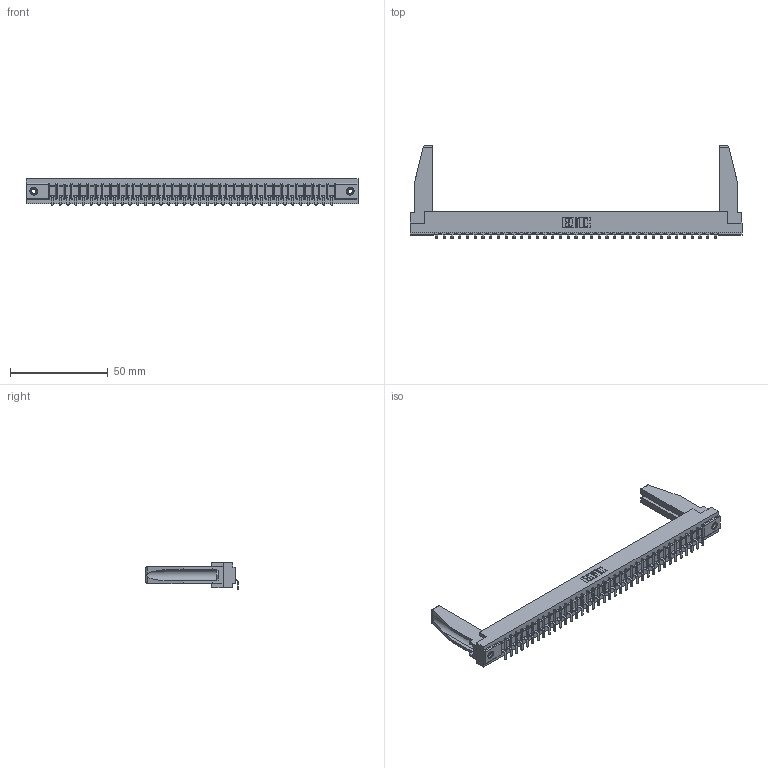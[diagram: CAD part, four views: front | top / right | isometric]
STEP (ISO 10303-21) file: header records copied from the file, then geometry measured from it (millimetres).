
FILE_DESCRIPTION (( 'STEP AP203' ), '1' );
FILE_NAME ('307-037-453-178.STEP', '2020-09-29T04:29:16', ( '' ), ( '' ), 'SwSTEP 2.0', 'SolidWorks 2020', '' );
FILE_SCHEMA (( 'CONFIG_CONTROL_DESIGN' ));
Length unit declared in the file: inch
Products named in the file (5): 307-290-002_553; 307 Part_.156 Dia Mounting Holes; 307-037-453-178; 345-250-001_345-250-001-102; 307-220-078
Assembly tree (42 placements, depth 2):
  307-037-453-178
    307 Part_.156 Dia Mounting Holes
    307-290-002_553  x37
    307-220-078  x2
    345-250-001_345-250-001-102  x2
Bounding box: 169.62 x 47.03 x 13.5 mm (x, y, z)
Volume: 22107.5 mm3; surface area: 26485.7 mm2
Topology: 42 solids, 42 shells, 3172 faces, 9681 edges, 6342 vertices
Faces by surface type: plane 1893, cylinder 1187, sphere 76, cone 12, torus 4
Entity records: 35629 total; most frequent: CARTESIAN_POINT 6010, ORIENTED_EDGE 5956, DIRECTION 5798, EDGE_CURVE 2978, LINE 2282, VECTOR 2282, VERTEX_POINT 1928, AXIS2_PLACEMENT_3D 1758
